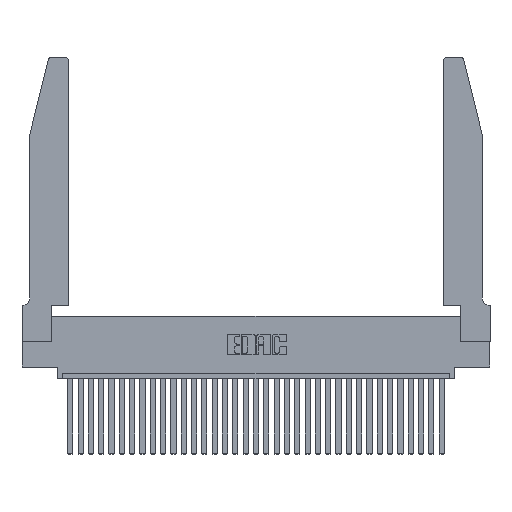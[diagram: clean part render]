
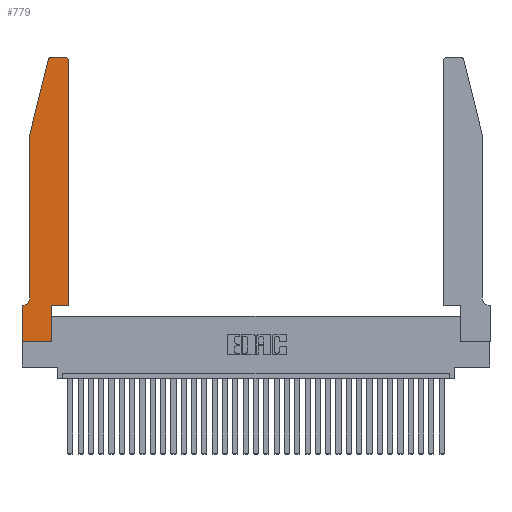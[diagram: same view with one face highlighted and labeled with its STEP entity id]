
A CAD part, top view. The second image highlights one B-rep face of the part: STEP entity #779.
In plain terms, the highlighted planar face has unit normal (0, 0, 1).
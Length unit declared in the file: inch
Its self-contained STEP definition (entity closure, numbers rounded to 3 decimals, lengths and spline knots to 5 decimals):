
#304 = CARTESIAN_POINT ( 'NONE',  ( 0., 0., 0.37 ) ) ;
#779 = ADVANCED_FACE ( 'NONE', ( #26643 ), #32462, .T. ) ;
#2028 = VECTOR ( 'NONE', #6424, 39.37008 ) ;
#2033 = CARTESIAN_POINT ( 'NONE',  ( 0.4505, 0.35, 0.37 ) ) ;
#2934 = CARTESIAN_POINT ( 'NONE',  ( 0.0755, 2., 0.37 ) ) ;
#3202 = LINE ( 'NONE', #2033, #14846 ) ;
#3963 = DIRECTION ( 'NONE',  ( 0., 0., 1. ) ) ;
#4713 = EDGE_CURVE ( 'NONE', #31097, #23450, #32574, .T. ) ;
#4857 = ORIENTED_EDGE ( 'NONE', *, *, #6323, .T. ) ;
#5622 = CARTESIAN_POINT ( 'NONE',  ( 0.0755, 0.42, 0.37 ) ) ;
#5889 = CARTESIAN_POINT ( 'NONE',  ( 0.4205, 2.72, 0.37 ) ) ;
#5898 = ORIENTED_EDGE ( 'NONE', *, *, #30140, .T. ) ;
#6050 = AXIS2_PLACEMENT_3D ( 'NONE', #7609, #7402, #25641 ) ;
#6204 = CARTESIAN_POINT ( 'NONE',  ( 0.2605, 2.75, 0.37 ) ) ;
#6266 = EDGE_CURVE ( 'NONE', #13213, #16792, #29207, .T. ) ;
#6323 = EDGE_CURVE ( 'NONE', #10448, #31097, #7120, .T. ) ;
#6424 = DIRECTION ( 'NONE',  ( -1., 0., 0. ) ) ;
#7120 = CIRCLE ( 'NONE', #23371, 0.03 ) ;
#7257 = CARTESIAN_POINT ( 'NONE',  ( 0.25487, 2.72718, 0.37 ) ) ;
#7349 = ORIENTED_EDGE ( 'NONE', *, *, #31785, .T. ) ;
#7402 = DIRECTION ( 'NONE',  ( 0., 0., 1. ) ) ;
#7609 = CARTESIAN_POINT ( 'NONE',  ( 0., 0.35, 0.37 ) ) ;
#8022 = ORIENTED_EDGE ( 'NONE', *, *, #15909, .T. ) ;
#8191 = DIRECTION ( 'NONE',  ( 1., 0., 0. ) ) ;
#8334 = CARTESIAN_POINT ( 'NONE',  ( 0.4205, 2.75, 0.37 ) ) ;
#8345 = ORIENTED_EDGE ( 'NONE', *, *, #4713, .T. ) ;
#8705 = EDGE_LOOP ( 'NONE', ( #5898, #4857, #8345, #8022, #21731, #11597, #7349, #15129, #27213, #32057, #24695, #14097 ) ) ;
#9725 = CARTESIAN_POINT ( 'NONE',  ( 0.0755, 0.35, 0.37 ) ) ;
#9763 = CARTESIAN_POINT ( 'NONE',  ( 0.284, 2.75, 0.37 ) ) ;
#9772 = CARTESIAN_POINT ( 'NONE',  ( 0.2865, 0., 0.37 ) ) ;
#10245 = CARTESIAN_POINT ( 'NONE',  ( 0.0755, 2., 0.37 ) ) ;
#10410 = VECTOR ( 'NONE', #12930, 39.37008 ) ;
#10448 = VERTEX_POINT ( 'NONE', #9763 ) ;
#10558 = DIRECTION ( 'NONE',  ( 0., -1., 0. ) ) ;
#11530 = EDGE_CURVE ( 'NONE', #26669, #13213, #17809, .T. ) ;
#11597 = ORIENTED_EDGE ( 'NONE', *, *, #6266, .T. ) ;
#11668 = VERTEX_POINT ( 'NONE', #8334 ) ;
#11766 = VECTOR ( 'NONE', #29069, 39.37008 ) ;
#11978 = VECTOR ( 'NONE', #27318, 39.37008 ) ;
#12062 = CARTESIAN_POINT ( 'NONE',  ( 0.0755, 2., 0.37 ) ) ;
#12317 = LINE ( 'NONE', #29764, #26001 ) ;
#12696 = CARTESIAN_POINT ( 'NONE',  ( 0.2865, 0.35, 0.37 ) ) ;
#12930 = DIRECTION ( 'NONE',  ( -0.239, -0.971, 0. ) ) ;
#13213 = VERTEX_POINT ( 'NONE', #24671 ) ;
#14097 = ORIENTED_EDGE ( 'NONE', *, *, #23148, .T. ) ;
#14506 = DIRECTION ( 'NONE',  ( 1., 0., 0. ) ) ;
#14846 = VECTOR ( 'NONE', #19964, 39.37008 ) ;
#15129 = ORIENTED_EDGE ( 'NONE', *, *, #26678, .T. ) ;
#15643 = EDGE_CURVE ( 'NONE', #18424, #17177, #27704, .T. ) ;
#15909 = EDGE_CURVE ( 'NONE', #23450, #26669, #27052, .T. ) ;
#16068 = CARTESIAN_POINT ( 'NONE',  ( 0.4505, 0.35, 0.37 ) ) ;
#16480 = CARTESIAN_POINT ( 'NONE',  ( 0.4505, 0.35, 0.37 ) ) ;
#16792 = VERTEX_POINT ( 'NONE', #17159 ) ;
#17159 = CARTESIAN_POINT ( 'NONE',  ( 0., 0.35, 0.37 ) ) ;
#17177 = VERTEX_POINT ( 'NONE', #16068 ) ;
#17756 = DIRECTION ( 'NONE',  ( 0., 1., 0. ) ) ;
#17809 = CIRCLE ( 'NONE', #25243, 0.07 ) ;
#17851 = VERTEX_POINT ( 'NONE', #304 ) ;
#18289 = EDGE_CURVE ( 'NONE', #17177, #29335, #3202, .T. ) ;
#18424 = VERTEX_POINT ( 'NONE', #12696 ) ;
#18585 = CARTESIAN_POINT ( 'NONE',  ( 0.4505, 2.72, 0.37 ) ) ;
#18899 = DIRECTION ( 'NONE',  ( 0., 0., 1. ) ) ;
#19153 = VECTOR ( 'NONE', #32143, 39.37008 ) ;
#19779 = DIRECTION ( 'NONE',  ( -1., 0., 0. ) ) ;
#19964 = DIRECTION ( 'NONE',  ( 0., 1., 0. ) ) ;
#20403 = CARTESIAN_POINT ( 'NONE',  ( 0.284, 2.72, 0.37 ) ) ;
#21495 = DIRECTION ( 'NONE',  ( 1., 0., 0. ) ) ;
#21513 = CIRCLE ( 'NONE', #31900, 0.03 ) ;
#21731 = ORIENTED_EDGE ( 'NONE', *, *, #11530, .T. ) ;
#23148 = EDGE_CURVE ( 'NONE', #29335, #11668, #21513, .T. ) ;
#23371 = AXIS2_PLACEMENT_3D ( 'NONE', #20403, #3963, #14506 ) ;
#23450 = VERTEX_POINT ( 'NONE', #10245 ) ;
#23623 = CARTESIAN_POINT ( 'NONE',  ( 0., 0., 0.37 ) ) ;
#24671 = CARTESIAN_POINT ( 'NONE',  ( 0.0055, 0.35, 0.37 ) ) ;
#24695 = ORIENTED_EDGE ( 'NONE', *, *, #18289, .T. ) ;
#25243 = AXIS2_PLACEMENT_3D ( 'NONE', #29777, #32583, #19779 ) ;
#25641 = DIRECTION ( 'NONE',  ( 1., 0., 0. ) ) ;
#25766 = VECTOR ( 'NONE', #8191, 39.37008 ) ;
#25794 = CARTESIAN_POINT ( 'NONE',  ( 0., 0., 0.37 ) ) ;
#26001 = VECTOR ( 'NONE', #17756, 39.37008 ) ;
#26552 = LINE ( 'NONE', #23623, #25766 ) ;
#26643 = FACE_OUTER_BOUND ( 'NONE', #8705, .T. ) ;
#26669 = VERTEX_POINT ( 'NONE', #5622 ) ;
#26678 = EDGE_CURVE ( 'NONE', #17851, #28988, #26552, .T. ) ;
#27052 = LINE ( 'NONE', #2934, #11766 ) ;
#27213 = ORIENTED_EDGE ( 'NONE', *, *, #32341, .T. ) ;
#27270 = VECTOR ( 'NONE', #10558, 39.37008 ) ;
#27318 = DIRECTION ( 'NONE',  ( 1., 0., 0. ) ) ;
#27704 = LINE ( 'NONE', #16480, #11978 ) ;
#28410 = LINE ( 'NONE', #25794, #27270 ) ;
#28988 = VERTEX_POINT ( 'NONE', #9772 ) ;
#29069 = DIRECTION ( 'NONE',  ( 0., -1., 0. ) ) ;
#29207 = LINE ( 'NONE', #9725, #19153 ) ;
#29335 = VERTEX_POINT ( 'NONE', #18585 ) ;
#29764 = CARTESIAN_POINT ( 'NONE',  ( 0.2865, 0.35, 0.37 ) ) ;
#29777 = CARTESIAN_POINT ( 'NONE',  ( 0.0055, 0.42, 0.37 ) ) ;
#30140 = EDGE_CURVE ( 'NONE', #11668, #10448, #31286, .T. ) ;
#31097 = VERTEX_POINT ( 'NONE', #7257 ) ;
#31286 = LINE ( 'NONE', #6204, #2028 ) ;
#31785 = EDGE_CURVE ( 'NONE', #16792, #17851, #28410, .T. ) ;
#31900 = AXIS2_PLACEMENT_3D ( 'NONE', #5889, #18899, #21495 ) ;
#32057 = ORIENTED_EDGE ( 'NONE', *, *, #15643, .T. ) ;
#32143 = DIRECTION ( 'NONE',  ( -1., 0., 0. ) ) ;
#32341 = EDGE_CURVE ( 'NONE', #28988, #18424, #12317, .T. ) ;
#32462 = PLANE ( 'NONE',  #6050 ) ;
#32574 = LINE ( 'NONE', #12062, #10410 ) ;
#32583 = DIRECTION ( 'NONE',  ( 0., 0., -1. ) ) ;
